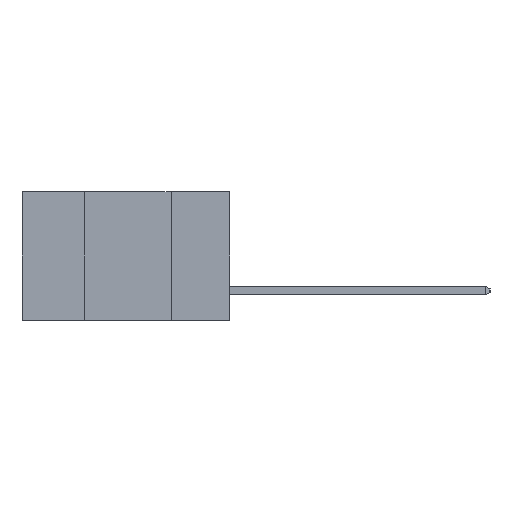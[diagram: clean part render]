
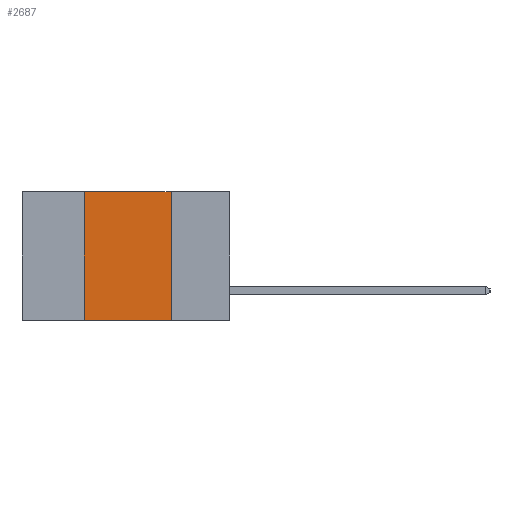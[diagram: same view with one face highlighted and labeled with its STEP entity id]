
A CAD part, left-side view. The second image highlights one B-rep face of the part: STEP entity #2687.
In plain terms, the highlighted planar face has unit normal (-1, 0, 0).
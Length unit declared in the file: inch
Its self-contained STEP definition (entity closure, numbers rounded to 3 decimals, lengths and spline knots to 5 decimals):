
#555 = VERTEX_POINT ( 'NONE', #8825 ) ;
#1066 = DIRECTION ( 'NONE',  ( 0., 0., -1. ) ) ;
#1146 = CARTESIAN_POINT ( 'NONE',  ( 0., 0.6, 0. ) ) ;
#1170 = VERTEX_POINT ( 'NONE', #11824 ) ;
#1475 = VECTOR ( 'NONE', #11010, 39.37008 ) ;
#1561 = EDGE_CURVE ( 'NONE', #11796, #1170, #6630, .T. ) ;
#1798 = FACE_OUTER_BOUND ( 'NONE', #10512, .T. ) ;
#1928 = DIRECTION ( 'NONE',  ( 1., 0., 0. ) ) ;
#2313 = ORIENTED_EDGE ( 'NONE', *, *, #2878, .F. ) ;
#2687 = ADVANCED_FACE ( 'NONE', ( #1798 ), #8541, .F. ) ;
#2878 = EDGE_CURVE ( 'NONE', #11796, #555, #4865, .T. ) ;
#3149 = EDGE_CURVE ( 'NONE', #555, #3446, #4403, .T. ) ;
#3175 = DIRECTION ( 'NONE',  ( 0., 0., -1. ) ) ;
#3340 = ORIENTED_EDGE ( 'NONE', *, *, #3149, .F. ) ;
#3446 = VERTEX_POINT ( 'NONE', #7380 ) ;
#4403 = LINE ( 'NONE', #10916, #1475 ) ;
#4865 = LINE ( 'NONE', #9898, #7044 ) ;
#5719 = EDGE_CURVE ( 'NONE', #3446, #1170, #8241, .T. ) ;
#6399 = ORIENTED_EDGE ( 'NONE', *, *, #1561, .T. ) ;
#6576 = ORIENTED_EDGE ( 'NONE', *, *, #5719, .F. ) ;
#6630 = LINE ( 'NONE', #8692, #8714 ) ;
#7044 = VECTOR ( 'NONE', #9705, 39.37008 ) ;
#7380 = CARTESIAN_POINT ( 'NONE',  ( 0., 0.17, 0. ) ) ;
#7736 = CARTESIAN_POINT ( 'NONE',  ( 0., 0.17, -0.37 ) ) ;
#7942 = VECTOR ( 'NONE', #1066, 39.37008 ) ;
#8241 = LINE ( 'NONE', #7736, #7942 ) ;
#8541 = PLANE ( 'NONE',  #10136 ) ;
#8620 = DIRECTION ( 'NONE',  ( 0., -1., 0. ) ) ;
#8692 = CARTESIAN_POINT ( 'NONE',  ( 0., 0.6, -0.37 ) ) ;
#8714 = VECTOR ( 'NONE', #8620, 39.37008 ) ;
#8825 = CARTESIAN_POINT ( 'NONE',  ( 0., 0.42, 0. ) ) ;
#8864 = CARTESIAN_POINT ( 'NONE',  ( 0., 0.42, -0.37 ) ) ;
#9705 = DIRECTION ( 'NONE',  ( 0., 0., 1. ) ) ;
#9898 = CARTESIAN_POINT ( 'NONE',  ( 0., 0.42, -0.37 ) ) ;
#10136 = AXIS2_PLACEMENT_3D ( 'NONE', #1146, #1928, #3175 ) ;
#10512 = EDGE_LOOP ( 'NONE', ( #6576, #3340, #2313, #6399 ) ) ;
#10916 = CARTESIAN_POINT ( 'NONE',  ( 0., 0.6, 0. ) ) ;
#11010 = DIRECTION ( 'NONE',  ( 0., -1., 0. ) ) ;
#11796 = VERTEX_POINT ( 'NONE', #8864 ) ;
#11824 = CARTESIAN_POINT ( 'NONE',  ( 0., 0.17, -0.37 ) ) ;
